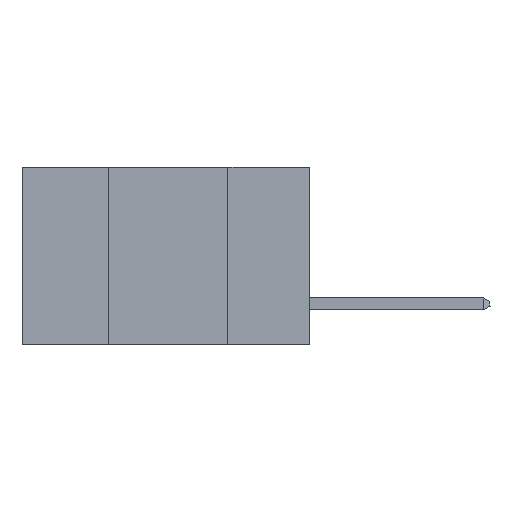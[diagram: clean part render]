
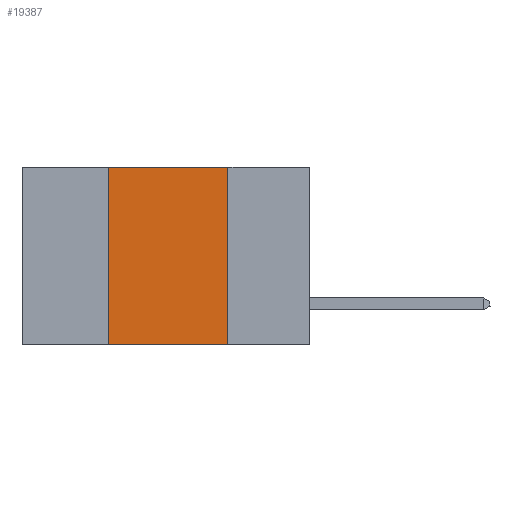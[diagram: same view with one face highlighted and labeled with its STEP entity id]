
A CAD part, left-side view. The second image highlights one B-rep face of the part: STEP entity #19387.
In plain terms, the highlighted planar face has unit normal (-1, 0, 0).
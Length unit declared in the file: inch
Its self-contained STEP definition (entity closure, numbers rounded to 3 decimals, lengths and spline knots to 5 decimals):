
#890 = CARTESIAN_POINT ( 'NONE',  ( 0., 0.6, -0.37 ) ) ;
#1042 = AXIS2_PLACEMENT_3D ( 'NONE', #9538, #21230, #13482 ) ;
#1130 = ORIENTED_EDGE ( 'NONE', *, *, #10255, .T. ) ;
#1277 = VECTOR ( 'NONE', #2078, 39.37008 ) ;
#2078 = DIRECTION ( 'NONE',  ( 0., -1., 0. ) ) ;
#3415 = CARTESIAN_POINT ( 'NONE',  ( 0., 0.42, -0.37 ) ) ;
#3498 = EDGE_CURVE ( 'NONE', #13642, #7516, #19037, .T. ) ;
#3648 = LINE ( 'NONE', #21831, #24036 ) ;
#3881 = DIRECTION ( 'NONE',  ( 0., -1., 0. ) ) ;
#4816 = DIRECTION ( 'NONE',  ( 0., 0., 1. ) ) ;
#6460 = CARTESIAN_POINT ( 'NONE',  ( 0., 0.17, 0. ) ) ;
#7067 = EDGE_LOOP ( 'NONE', ( #25048, #16062, #21416, #1130 ) ) ;
#7260 = VECTOR ( 'NONE', #20372, 39.37008 ) ;
#7516 = VERTEX_POINT ( 'NONE', #11080 ) ;
#9208 = PLANE ( 'NONE',  #1042 ) ;
#9538 = CARTESIAN_POINT ( 'NONE',  ( 0., 0.6, 0. ) ) ;
#10255 = EDGE_CURVE ( 'NONE', #22467, #7516, #16748, .T. ) ;
#11012 = VERTEX_POINT ( 'NONE', #17834 ) ;
#11080 = CARTESIAN_POINT ( 'NONE',  ( 0., 0.17, -0.37 ) ) ;
#11395 = FACE_OUTER_BOUND ( 'NONE', #7067, .T. ) ;
#11617 = CARTESIAN_POINT ( 'NONE',  ( 0., 0.17, 0. ) ) ;
#12389 = VECTOR ( 'NONE', #4816, 39.37008 ) ;
#13482 = DIRECTION ( 'NONE',  ( 0., 0., -1. ) ) ;
#13642 = VERTEX_POINT ( 'NONE', #11617 ) ;
#16062 = ORIENTED_EDGE ( 'NONE', *, *, #25525, .F. ) ;
#16748 = LINE ( 'NONE', #890, #1277 ) ;
#17834 = CARTESIAN_POINT ( 'NONE',  ( 0., 0.42, 0. ) ) ;
#19037 = LINE ( 'NONE', #6460, #7260 ) ;
#19387 = ADVANCED_FACE ( 'NONE', ( #11395 ), #9208, .F. ) ;
#20372 = DIRECTION ( 'NONE',  ( 0., 0., -1. ) ) ;
#20401 = LINE ( 'NONE', #22516, #12389 ) ;
#21230 = DIRECTION ( 'NONE',  ( 1., 0., 0. ) ) ;
#21416 = ORIENTED_EDGE ( 'NONE', *, *, #24093, .F. ) ;
#21831 = CARTESIAN_POINT ( 'NONE',  ( 0., 0.6, 0. ) ) ;
#22467 = VERTEX_POINT ( 'NONE', #3415 ) ;
#22516 = CARTESIAN_POINT ( 'NONE',  ( 0., 0.42, 0. ) ) ;
#24036 = VECTOR ( 'NONE', #3881, 39.37008 ) ;
#24093 = EDGE_CURVE ( 'NONE', #22467, #11012, #20401, .T. ) ;
#25048 = ORIENTED_EDGE ( 'NONE', *, *, #3498, .F. ) ;
#25525 = EDGE_CURVE ( 'NONE', #11012, #13642, #3648, .T. ) ;
